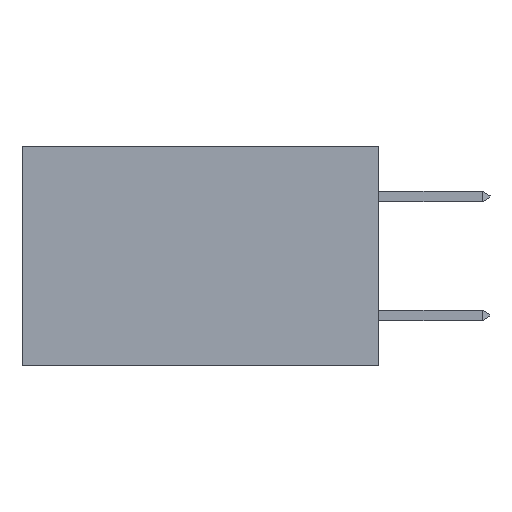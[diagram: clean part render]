
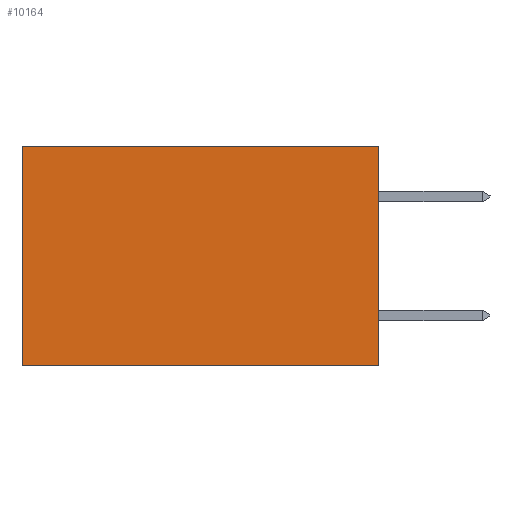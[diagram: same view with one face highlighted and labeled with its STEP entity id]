
A CAD part, left-side view. The second image highlights one B-rep face of the part: STEP entity #10164.
In plain terms, the highlighted planar face has unit normal (-1, 0, 0).
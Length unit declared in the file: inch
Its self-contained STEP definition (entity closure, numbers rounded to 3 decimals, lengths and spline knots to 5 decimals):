
#84 = DIRECTION ( 'NONE',  ( 0., 1., 0. ) ) ;
#638 = EDGE_CURVE ( 'NONE', #10519, #18333, #18215, .T. ) ;
#1805 = DIRECTION ( 'NONE',  ( 0., 0., -1. ) ) ;
#2220 = EDGE_CURVE ( 'NONE', #16152, #18425, #18725, .T. ) ;
#2424 = DIRECTION ( 'NONE',  ( 0., 0., -1. ) ) ;
#2429 = CARTESIAN_POINT ( 'NONE',  ( 0.2615, 0., 0. ) ) ;
#3966 = ORIENTED_EDGE ( 'NONE', *, *, #2220, .T. ) ;
#3983 = CARTESIAN_POINT ( 'NONE',  ( 0.2615, 0.6, -0.37 ) ) ;
#8250 = DIRECTION ( 'NONE',  ( 1., 0., 0. ) ) ;
#9203 = LINE ( 'NONE', #20465, #13282 ) ;
#9712 = DIRECTION ( 'NONE',  ( 0., 0., -1. ) ) ;
#9847 = CARTESIAN_POINT ( 'NONE',  ( 0.2615, 0.6, 0. ) ) ;
#10164 = ADVANCED_FACE ( 'NONE', ( #15174 ), #17357, .F. ) ;
#10519 = VERTEX_POINT ( 'NONE', #21752 ) ;
#11772 = CARTESIAN_POINT ( 'NONE',  ( 0.2615, 0., -0.37 ) ) ;
#11955 = ORIENTED_EDGE ( 'NONE', *, *, #17080, .T. ) ;
#12130 = VECTOR ( 'NONE', #1805, 39.37008 ) ;
#13010 = CARTESIAN_POINT ( 'NONE',  ( 0.2615, 0., -0.37 ) ) ;
#13282 = VECTOR ( 'NONE', #84, 39.37008 ) ;
#14356 = VECTOR ( 'NONE', #23031, 39.37008 ) ;
#15174 = FACE_OUTER_BOUND ( 'NONE', #20463, .T. ) ;
#15588 = LINE ( 'NONE', #2429, #14356 ) ;
#16152 = VERTEX_POINT ( 'NONE', #9847 ) ;
#16897 = VECTOR ( 'NONE', #2424, 39.37008 ) ;
#17080 = EDGE_CURVE ( 'NONE', #10519, #16152, #15588, .T. ) ;
#17357 = PLANE ( 'NONE',  #23053 ) ;
#18215 = LINE ( 'NONE', #13010, #12130 ) ;
#18333 = VERTEX_POINT ( 'NONE', #19379 ) ;
#18425 = VERTEX_POINT ( 'NONE', #20460 ) ;
#18725 = LINE ( 'NONE', #3983, #16897 ) ;
#19379 = CARTESIAN_POINT ( 'NONE',  ( 0.2615, 0., -0.37 ) ) ;
#19959 = EDGE_CURVE ( 'NONE', #18333, #18425, #9203, .T. ) ;
#20460 = CARTESIAN_POINT ( 'NONE',  ( 0.2615, 0.6, -0.37 ) ) ;
#20463 = EDGE_LOOP ( 'NONE', ( #3966, #20656, #20583, #11955 ) ) ;
#20465 = CARTESIAN_POINT ( 'NONE',  ( 0.2615, 0., -0.37 ) ) ;
#20583 = ORIENTED_EDGE ( 'NONE', *, *, #638, .F. ) ;
#20656 = ORIENTED_EDGE ( 'NONE', *, *, #19959, .F. ) ;
#21752 = CARTESIAN_POINT ( 'NONE',  ( 0.2615, 0., 0. ) ) ;
#23031 = DIRECTION ( 'NONE',  ( 0., 1., 0. ) ) ;
#23053 = AXIS2_PLACEMENT_3D ( 'NONE', #11772, #8250, #9712 ) ;
